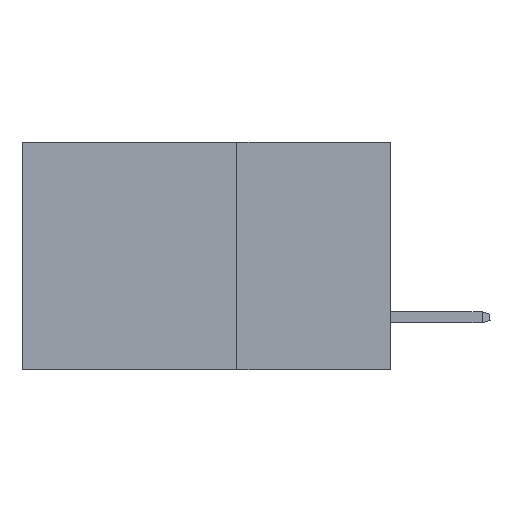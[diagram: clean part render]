
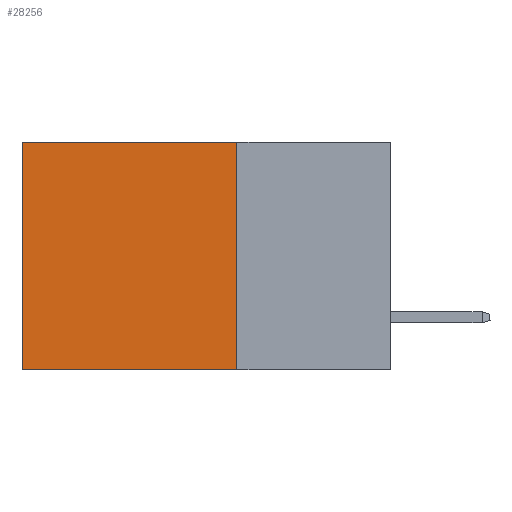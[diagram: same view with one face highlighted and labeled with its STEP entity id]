
A CAD part, left-side view. The second image highlights one B-rep face of the part: STEP entity #28256.
In plain terms, the highlighted planar face has unit normal (-1, 0, 0).
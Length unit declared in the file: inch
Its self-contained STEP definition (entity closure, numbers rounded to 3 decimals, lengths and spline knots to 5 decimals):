
#1422 = PLANE ( 'NONE',  #7151 ) ;
#2539 = ORIENTED_EDGE ( 'NONE', *, *, #13469, .F. ) ;
#2597 = DIRECTION ( 'NONE',  ( 0., 0., -1. ) ) ;
#2778 = VERTEX_POINT ( 'NONE', #34932 ) ;
#3320 = CARTESIAN_POINT ( 'NONE',  ( 0.2875, 0.6, 0. ) ) ;
#4400 = VERTEX_POINT ( 'NONE', #3320 ) ;
#5036 = VERTEX_POINT ( 'NONE', #18162 ) ;
#5563 = ORIENTED_EDGE ( 'NONE', *, *, #16552, .F. ) ;
#5675 = VECTOR ( 'NONE', #12510, 39.37008 ) ;
#6646 = CARTESIAN_POINT ( 'NONE',  ( 0.2875, 0.6, -0.37 ) ) ;
#7151 = AXIS2_PLACEMENT_3D ( 'NONE', #33130, #29746, #11589 ) ;
#8108 = EDGE_LOOP ( 'NONE', ( #12098, #5563, #2539, #12949 ) ) ;
#9517 = EDGE_CURVE ( 'NONE', #4400, #30794, #22705, .T. ) ;
#10214 = LINE ( 'NONE', #37786, #45679 ) ;
#11589 = DIRECTION ( 'NONE',  ( 0., 0., -1. ) ) ;
#12098 = ORIENTED_EDGE ( 'NONE', *, *, #9517, .T. ) ;
#12286 = EDGE_CURVE ( 'NONE', #5036, #4400, #10214, .T. ) ;
#12510 = DIRECTION ( 'NONE',  ( 0., 0., -1. ) ) ;
#12857 = LINE ( 'NONE', #33737, #5675 ) ;
#12949 = ORIENTED_EDGE ( 'NONE', *, *, #12286, .T. ) ;
#13469 = EDGE_CURVE ( 'NONE', #5036, #2778, #12857, .T. ) ;
#16552 = EDGE_CURVE ( 'NONE', #2778, #30794, #32318, .T. ) ;
#18162 = CARTESIAN_POINT ( 'NONE',  ( 0.2875, 0.25, 0. ) ) ;
#21036 = VECTOR ( 'NONE', #2597, 39.37008 ) ;
#22690 = FACE_OUTER_BOUND ( 'NONE', #8108, .T. ) ;
#22705 = LINE ( 'NONE', #23771, #21036 ) ;
#22713 = DIRECTION ( 'NONE',  ( 0., 1., 0. ) ) ;
#23507 = DIRECTION ( 'NONE',  ( 0., 1., 0. ) ) ;
#23771 = CARTESIAN_POINT ( 'NONE',  ( 0.2875, 0.6, 0. ) ) ;
#28256 = ADVANCED_FACE ( 'NONE', ( #22690 ), #1422, .F. ) ;
#29746 = DIRECTION ( 'NONE',  ( 1., 0., 0. ) ) ;
#30794 = VERTEX_POINT ( 'NONE', #6646 ) ;
#32318 = LINE ( 'NONE', #43945, #33459 ) ;
#33130 = CARTESIAN_POINT ( 'NONE',  ( 0.2875, 0.25, 0. ) ) ;
#33459 = VECTOR ( 'NONE', #22713, 39.37008 ) ;
#33737 = CARTESIAN_POINT ( 'NONE',  ( 0.2875, 0.25, 0. ) ) ;
#34932 = CARTESIAN_POINT ( 'NONE',  ( 0.2875, 0.25, -0.37 ) ) ;
#37786 = CARTESIAN_POINT ( 'NONE',  ( 0.2875, 0.25, 0. ) ) ;
#43945 = CARTESIAN_POINT ( 'NONE',  ( 0.2875, 0.25, -0.37 ) ) ;
#45679 = VECTOR ( 'NONE', #23507, 39.37008 ) ;
